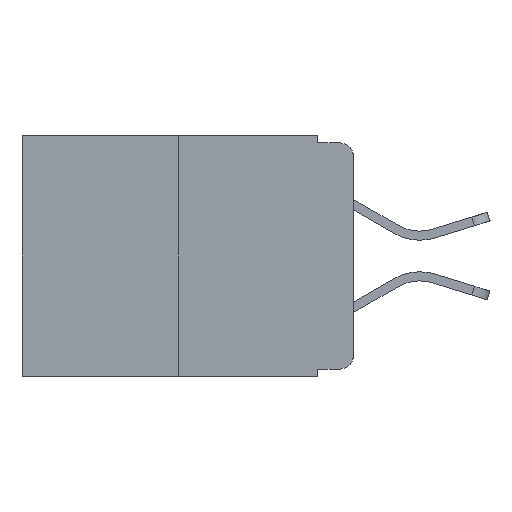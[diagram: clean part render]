
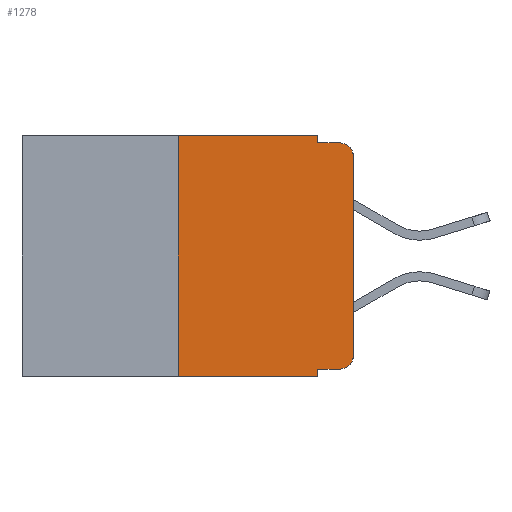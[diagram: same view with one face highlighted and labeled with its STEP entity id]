
A CAD part, left-side view. The second image highlights one B-rep face of the part: STEP entity #1278.
In plain terms, the highlighted planar face has unit normal (-1, 0, 0).
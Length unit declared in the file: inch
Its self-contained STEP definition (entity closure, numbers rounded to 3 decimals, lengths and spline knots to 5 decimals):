
#409 = VERTEX_POINT ( 'NONE', #1692 ) ;
#421 = LINE ( 'NONE', #13490, #11745 ) ;
#506 = LINE ( 'NONE', #3645, #12462 ) ;
#578 = EDGE_CURVE ( 'NONE', #6348, #3895, #421, .T. ) ;
#961 = VECTOR ( 'NONE', #5409, 39.37008 ) ;
#982 = DIRECTION ( 'NONE',  ( 0., 0., 1. ) ) ;
#1093 = CARTESIAN_POINT ( 'NONE',  ( 0., 0.051, 0. ) ) ;
#1278 = ADVANCED_FACE ( 'NONE', ( #4552 ), #9686, .F. ) ;
#1305 = EDGE_CURVE ( 'NONE', #1423, #8577, #1341, .T. ) ;
#1312 = DIRECTION ( 'NONE',  ( -1., 0., 0. ) ) ;
#1321 = DIRECTION ( 'NONE',  ( 0., 0., -1. ) ) ;
#1341 = LINE ( 'NONE', #12915, #961 ) ;
#1397 = EDGE_CURVE ( 'NONE', #11507, #1423, #13321, .T. ) ;
#1423 = VERTEX_POINT ( 'NONE', #14228 ) ;
#1692 = CARTESIAN_POINT ( 'NONE',  ( 0., 0.02, -0.333 ) ) ;
#1773 = ORIENTED_EDGE ( 'NONE', *, *, #3850, .T. ) ;
#1787 = LINE ( 'NONE', #5215, #10084 ) ;
#1897 = VECTOR ( 'NONE', #11142, 39.37008 ) ;
#2225 = EDGE_CURVE ( 'NONE', #8577, #3552, #12050, .T. ) ;
#2308 = LINE ( 'NONE', #12147, #1897 ) ;
#2426 = CARTESIAN_POINT ( 'NONE',  ( 0., 0.051, -0.01 ) ) ;
#2468 = CARTESIAN_POINT ( 'NONE',  ( 0., 0., -0.313 ) ) ;
#2507 = ORIENTED_EDGE ( 'NONE', *, *, #4626, .T. ) ;
#2948 = ORIENTED_EDGE ( 'NONE', *, *, #3031, .F. ) ;
#3031 = EDGE_CURVE ( 'NONE', #3552, #13553, #2308, .T. ) ;
#3056 = CARTESIAN_POINT ( 'NONE',  ( 0., 0.02, -0.03 ) ) ;
#3069 = ORIENTED_EDGE ( 'NONE', *, *, #2225, .F. ) ;
#3395 = CIRCLE ( 'NONE', #12692, 0.02 ) ;
#3521 = ORIENTED_EDGE ( 'NONE', *, *, #578, .F. ) ;
#3552 = VERTEX_POINT ( 'NONE', #2426 ) ;
#3645 = CARTESIAN_POINT ( 'NONE',  ( 0., 0.051, -0.333 ) ) ;
#3850 = EDGE_CURVE ( 'NONE', #13639, #13553, #7414, .T. ) ;
#3895 = VERTEX_POINT ( 'NONE', #6545 ) ;
#4105 = DIRECTION ( 'NONE',  ( 0., -1., 0. ) ) ;
#4256 = DIRECTION ( 'NONE',  ( 0., 0., -1. ) ) ;
#4552 = FACE_OUTER_BOUND ( 'NONE', #8107, .T. ) ;
#4626 = EDGE_CURVE ( 'NONE', #14278, #13639, #8221, .T. ) ;
#4879 = CARTESIAN_POINT ( 'NONE',  ( 0., 0.02, -0.01 ) ) ;
#5019 = CARTESIAN_POINT ( 'NONE',  ( 0., 0., -0.03 ) ) ;
#5215 = CARTESIAN_POINT ( 'NONE',  ( 0., 0.473, -0.343 ) ) ;
#5321 = CARTESIAN_POINT ( 'NONE',  ( 0., 0.25, -0.343 ) ) ;
#5357 = DIRECTION ( 'NONE',  ( 0., 0., -1. ) ) ;
#5409 = DIRECTION ( 'NONE',  ( 0., -1., 0. ) ) ;
#5874 = EDGE_CURVE ( 'NONE', #11507, #3895, #1787, .T. ) ;
#6348 = VERTEX_POINT ( 'NONE', #7075 ) ;
#6460 = AXIS2_PLACEMENT_3D ( 'NONE', #12833, #11848, #5357 ) ;
#6545 = CARTESIAN_POINT ( 'NONE',  ( 0., 0.051, -0.343 ) ) ;
#7021 = ORIENTED_EDGE ( 'NONE', *, *, #13561, .T. ) ;
#7053 = ORIENTED_EDGE ( 'NONE', *, *, #1305, .F. ) ;
#7075 = CARTESIAN_POINT ( 'NONE',  ( 0., 0.051, -0.333 ) ) ;
#7414 = CIRCLE ( 'NONE', #8930, 0.02 ) ;
#7620 = VECTOR ( 'NONE', #13148, 39.37008 ) ;
#7934 = ORIENTED_EDGE ( 'NONE', *, *, #5874, .T. ) ;
#8107 = EDGE_LOOP ( 'NONE', ( #2507, #1773, #2948, #3069, #7053, #11347, #7934, #3521, #12903, #7021 ) ) ;
#8154 = CARTESIAN_POINT ( 'NONE',  ( 0., 0.02, -0.313 ) ) ;
#8221 = LINE ( 'NONE', #11127, #13244 ) ;
#8577 = VERTEX_POINT ( 'NONE', #8999 ) ;
#8930 = AXIS2_PLACEMENT_3D ( 'NONE', #3056, #10844, #4256 ) ;
#8999 = CARTESIAN_POINT ( 'NONE',  ( 0., 0.051, 0. ) ) ;
#9040 = DIRECTION ( 'NONE',  ( 0., 0., -1. ) ) ;
#9268 = DIRECTION ( 'NONE',  ( 0., 0., -1. ) ) ;
#9686 = PLANE ( 'NONE',  #6460 ) ;
#10084 = VECTOR ( 'NONE', #4105, 39.37008 ) ;
#10265 = DIRECTION ( 'NONE',  ( 0., -1., 0. ) ) ;
#10844 = DIRECTION ( 'NONE',  ( -1., 0., 0. ) ) ;
#11127 = CARTESIAN_POINT ( 'NONE',  ( 0., 0., 0. ) ) ;
#11142 = DIRECTION ( 'NONE',  ( 0., -1., 0. ) ) ;
#11347 = ORIENTED_EDGE ( 'NONE', *, *, #1397, .F. ) ;
#11507 = VERTEX_POINT ( 'NONE', #5321 ) ;
#11745 = VECTOR ( 'NONE', #1321, 39.37008 ) ;
#11848 = DIRECTION ( 'NONE',  ( 1., 0., 0. ) ) ;
#12050 = LINE ( 'NONE', #1093, #14453 ) ;
#12124 = CARTESIAN_POINT ( 'NONE',  ( 0., 0.25, 0. ) ) ;
#12147 = CARTESIAN_POINT ( 'NONE',  ( 0., 0.051, -0.01 ) ) ;
#12462 = VECTOR ( 'NONE', #10265, 39.37008 ) ;
#12692 = AXIS2_PLACEMENT_3D ( 'NONE', #8154, #1312, #9268 ) ;
#12833 = CARTESIAN_POINT ( 'NONE',  ( 0., 0.473, 0. ) ) ;
#12903 = ORIENTED_EDGE ( 'NONE', *, *, #14246, .T. ) ;
#12915 = CARTESIAN_POINT ( 'NONE',  ( 0., 0.473, 0. ) ) ;
#13148 = DIRECTION ( 'NONE',  ( 0., 0., 1. ) ) ;
#13244 = VECTOR ( 'NONE', #982, 39.37008 ) ;
#13321 = LINE ( 'NONE', #12124, #7620 ) ;
#13490 = CARTESIAN_POINT ( 'NONE',  ( 0., 0.051, 0. ) ) ;
#13553 = VERTEX_POINT ( 'NONE', #4879 ) ;
#13561 = EDGE_CURVE ( 'NONE', #409, #14278, #3395, .T. ) ;
#13639 = VERTEX_POINT ( 'NONE', #5019 ) ;
#14228 = CARTESIAN_POINT ( 'NONE',  ( 0., 0.25, 0. ) ) ;
#14246 = EDGE_CURVE ( 'NONE', #6348, #409, #506, .T. ) ;
#14278 = VERTEX_POINT ( 'NONE', #2468 ) ;
#14453 = VECTOR ( 'NONE', #9040, 39.37008 ) ;
